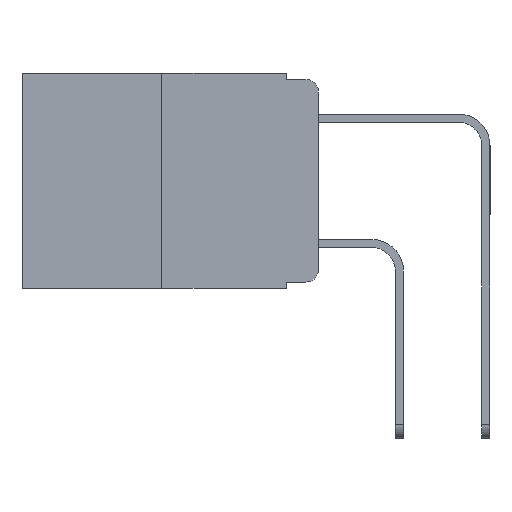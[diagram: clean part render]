
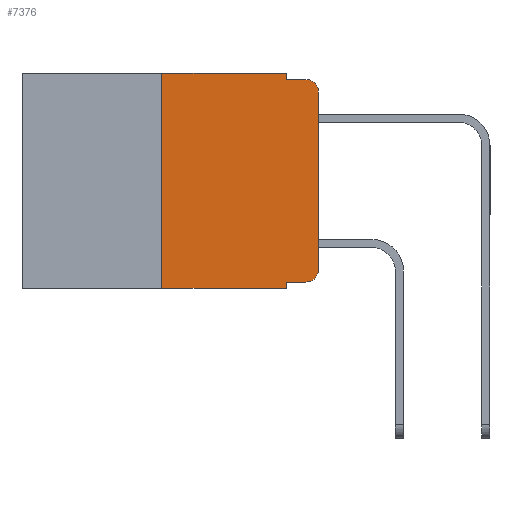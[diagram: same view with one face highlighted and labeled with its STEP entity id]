
A CAD part, left-side view. The second image highlights one B-rep face of the part: STEP entity #7376.
In plain terms, the highlighted planar face has unit normal (-1, 0, 0).
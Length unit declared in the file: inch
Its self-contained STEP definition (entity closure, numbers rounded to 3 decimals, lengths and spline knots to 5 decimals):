
#425 = LINE ( 'NONE', #3407, #15561 ) ;
#507 = VERTEX_POINT ( 'NONE', #9171 ) ;
#1260 = CARTESIAN_POINT ( 'NONE',  ( 0., 0., -0.03 ) ) ;
#1827 = DIRECTION ( 'NONE',  ( 0., -1., 0. ) ) ;
#1957 = LINE ( 'NONE', #12849, #9427 ) ;
#2116 = CARTESIAN_POINT ( 'NONE',  ( 0., 0.051, 0. ) ) ;
#2167 = VERTEX_POINT ( 'NONE', #5614 ) ;
#2322 = VECTOR ( 'NONE', #18113, 39.37008 ) ;
#2574 = FACE_OUTER_BOUND ( 'NONE', #15544, .T. ) ;
#2700 = VERTEX_POINT ( 'NONE', #14198 ) ;
#3300 = DIRECTION ( 'NONE',  ( 0., -1., 0. ) ) ;
#3320 = EDGE_CURVE ( 'NONE', #4076, #2700, #7911, .T. ) ;
#3407 = CARTESIAN_POINT ( 'NONE',  ( 0., 0.25, 0. ) ) ;
#3709 = VERTEX_POINT ( 'NONE', #14906 ) ;
#4076 = VERTEX_POINT ( 'NONE', #4242 ) ;
#4097 = CARTESIAN_POINT ( 'NONE',  ( 0., 0.051, 0. ) ) ;
#4195 = DIRECTION ( 'NONE',  ( 0., 0., 1. ) ) ;
#4242 = CARTESIAN_POINT ( 'NONE',  ( 0., 0.02, -0.333 ) ) ;
#4339 = EDGE_CURVE ( 'NONE', #14114, #4076, #14568, .T. ) ;
#5212 = LINE ( 'NONE', #10710, #16611 ) ;
#5353 = EDGE_CURVE ( 'NONE', #14114, #507, #6930, .T. ) ;
#5614 = CARTESIAN_POINT ( 'NONE',  ( 0., 0.02, -0.01 ) ) ;
#5986 = DIRECTION ( 'NONE',  ( 0., -1., 0. ) ) ;
#6000 = ORIENTED_EDGE ( 'NONE', *, *, #11169, .T. ) ;
#6356 = EDGE_CURVE ( 'NONE', #3709, #11791, #425, .T. ) ;
#6373 = DIRECTION ( 'NONE',  ( 0., 0., 1. ) ) ;
#6583 = DIRECTION ( 'NONE',  ( -1., 0., 0. ) ) ;
#6886 = CARTESIAN_POINT ( 'NONE',  ( 0., 0.051, -0.333 ) ) ;
#6930 = LINE ( 'NONE', #8230, #17810 ) ;
#7318 = EDGE_CURVE ( 'NONE', #16123, #11557, #17959, .T. ) ;
#7376 = ADVANCED_FACE ( 'NONE', ( #2574 ), #12953, .F. ) ;
#7506 = ORIENTED_EDGE ( 'NONE', *, *, #6356, .F. ) ;
#7776 = ORIENTED_EDGE ( 'NONE', *, *, #5353, .F. ) ;
#7880 = CIRCLE ( 'NONE', #13413, 0.02 ) ;
#7911 = CIRCLE ( 'NONE', #18395, 0.02 ) ;
#7992 = ORIENTED_EDGE ( 'NONE', *, *, #4339, .T. ) ;
#8230 = CARTESIAN_POINT ( 'NONE',  ( 0., 0.051, 0. ) ) ;
#8292 = EDGE_CURVE ( 'NONE', #11557, #2167, #13985, .T. ) ;
#8305 = ORIENTED_EDGE ( 'NONE', *, *, #3320, .T. ) ;
#8390 = ORIENTED_EDGE ( 'NONE', *, *, #8292, .F. ) ;
#8450 = DIRECTION ( 'NONE',  ( -1., 0., 0. ) ) ;
#8555 = VERTEX_POINT ( 'NONE', #1260 ) ;
#8718 = DIRECTION ( 'NONE',  ( 1., 0., 0. ) ) ;
#9105 = ORIENTED_EDGE ( 'NONE', *, *, #13923, .T. ) ;
#9171 = CARTESIAN_POINT ( 'NONE',  ( 0., 0.051, -0.343 ) ) ;
#9184 = CARTESIAN_POINT ( 'NONE',  ( 0., 0.473, 0. ) ) ;
#9427 = VECTOR ( 'NONE', #4195, 39.37008 ) ;
#9632 = CARTESIAN_POINT ( 'NONE',  ( 0., 0.051, -0.01 ) ) ;
#10211 = EDGE_CURVE ( 'NONE', #8555, #2167, #7880, .T. ) ;
#10710 = CARTESIAN_POINT ( 'NONE',  ( 0., 0.473, -0.343 ) ) ;
#10795 = VECTOR ( 'NONE', #5986, 39.37008 ) ;
#11169 = EDGE_CURVE ( 'NONE', #2700, #8555, #1957, .T. ) ;
#11512 = CARTESIAN_POINT ( 'NONE',  ( 0., 0.473, 0. ) ) ;
#11557 = VERTEX_POINT ( 'NONE', #15149 ) ;
#11791 = VERTEX_POINT ( 'NONE', #18768 ) ;
#12849 = CARTESIAN_POINT ( 'NONE',  ( 0., 0., 0. ) ) ;
#12953 = PLANE ( 'NONE',  #13478 ) ;
#12997 = ORIENTED_EDGE ( 'NONE', *, *, #10211, .T. ) ;
#13219 = EDGE_CURVE ( 'NONE', #11791, #16123, #18221, .T. ) ;
#13413 = AXIS2_PLACEMENT_3D ( 'NONE', #15121, #6583, #16519 ) ;
#13478 = AXIS2_PLACEMENT_3D ( 'NONE', #11512, #8718, #18633 ) ;
#13923 = EDGE_CURVE ( 'NONE', #3709, #507, #5212, .T. ) ;
#13985 = LINE ( 'NONE', #9632, #2322 ) ;
#14114 = VERTEX_POINT ( 'NONE', #6886 ) ;
#14198 = CARTESIAN_POINT ( 'NONE',  ( 0., 0., -0.313 ) ) ;
#14203 = VECTOR ( 'NONE', #17087, 39.37008 ) ;
#14568 = LINE ( 'NONE', #17383, #10795 ) ;
#14906 = CARTESIAN_POINT ( 'NONE',  ( 0., 0.25, -0.343 ) ) ;
#15121 = CARTESIAN_POINT ( 'NONE',  ( 0., 0.02, -0.03 ) ) ;
#15149 = CARTESIAN_POINT ( 'NONE',  ( 0., 0.051, -0.01 ) ) ;
#15544 = EDGE_LOOP ( 'NONE', ( #6000, #12997, #8390, #16159, #15859, #7506, #9105, #7776, #7992, #8305 ) ) ;
#15561 = VECTOR ( 'NONE', #6373, 39.37008 ) ;
#15859 = ORIENTED_EDGE ( 'NONE', *, *, #13219, .F. ) ;
#16123 = VERTEX_POINT ( 'NONE', #2116 ) ;
#16159 = ORIENTED_EDGE ( 'NONE', *, *, #7318, .F. ) ;
#16519 = DIRECTION ( 'NONE',  ( 0., 0., -1. ) ) ;
#16611 = VECTOR ( 'NONE', #1827, 39.37008 ) ;
#16726 = DIRECTION ( 'NONE',  ( 0., 0., -1. ) ) ;
#16941 = CARTESIAN_POINT ( 'NONE',  ( 0., 0.02, -0.313 ) ) ;
#17087 = DIRECTION ( 'NONE',  ( 0., 0., -1. ) ) ;
#17383 = CARTESIAN_POINT ( 'NONE',  ( 0., 0.051, -0.333 ) ) ;
#17764 = VECTOR ( 'NONE', #3300, 39.37008 ) ;
#17810 = VECTOR ( 'NONE', #16726, 39.37008 ) ;
#17959 = LINE ( 'NONE', #4097, #14203 ) ;
#18113 = DIRECTION ( 'NONE',  ( 0., -1., 0. ) ) ;
#18221 = LINE ( 'NONE', #9184, #17764 ) ;
#18366 = DIRECTION ( 'NONE',  ( 0., 0., -1. ) ) ;
#18395 = AXIS2_PLACEMENT_3D ( 'NONE', #16941, #8450, #18366 ) ;
#18633 = DIRECTION ( 'NONE',  ( 0., 0., -1. ) ) ;
#18768 = CARTESIAN_POINT ( 'NONE',  ( 0., 0.25, 0. ) ) ;
